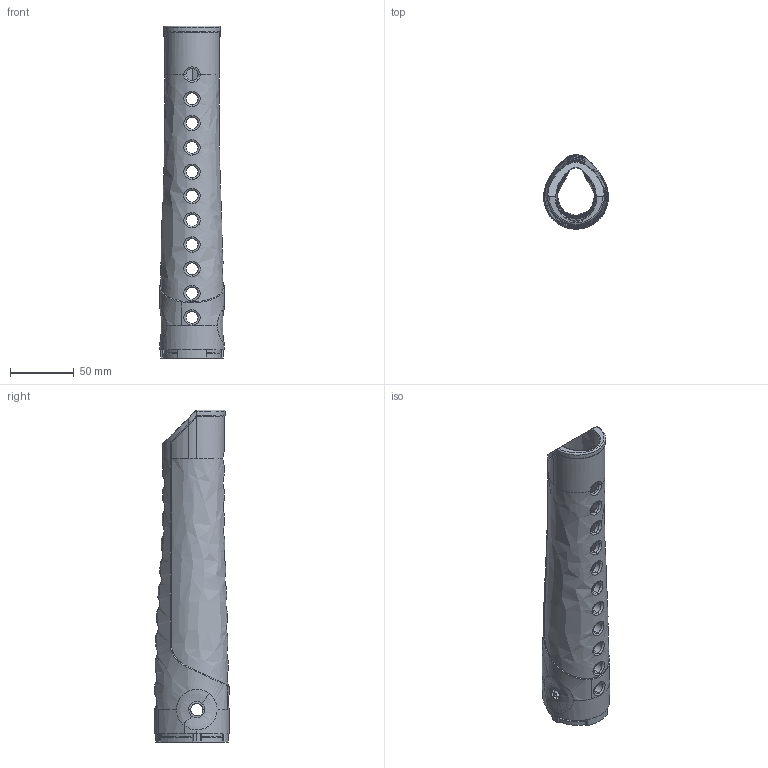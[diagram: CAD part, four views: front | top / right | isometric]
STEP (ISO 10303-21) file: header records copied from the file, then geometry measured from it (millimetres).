
FILE_DESCRIPTION (( 'STEP AP203' ), '1' );
FILE_NAME ('Orca Handguard Mid V5.3.1.STEP', '2023-01-20T23:42:40', ( '' ), ( '' ), 'SwSTEP 2.0', 'SolidWorks 2021', '' );
FILE_SCHEMA (( 'CONFIG_CONTROL_DESIGN' ));
Length unit declared in the file: inch
Products named in the file (1): Orca Handguard Mid V5.3.1
Bounding box: 50.8 x 58.26 x 260.35 mm (x, y, z)
Volume: 230707.9 mm3; surface area: 70527.2 mm2
Topology: 1 solids, 1 shells, 356 faces, 1094 edges, 706 vertices
Faces by surface type: bspline 179, cylinder 87, plane 50, sphere 36, torus 4
Entity records: 41074 total; most frequent: CARTESIAN_POINT 33347, ORIENTED_EDGE 2044, EDGE_CURVE 1022, DIRECTION 924, VERTEX_POINT 658, B_SPLINE_CURVE_WITH_KNOTS 617, EDGE_LOOP 394, ADVANCED_FACE 356
